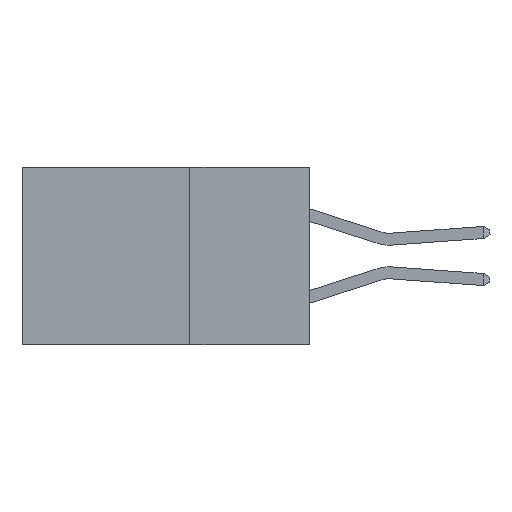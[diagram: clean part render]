
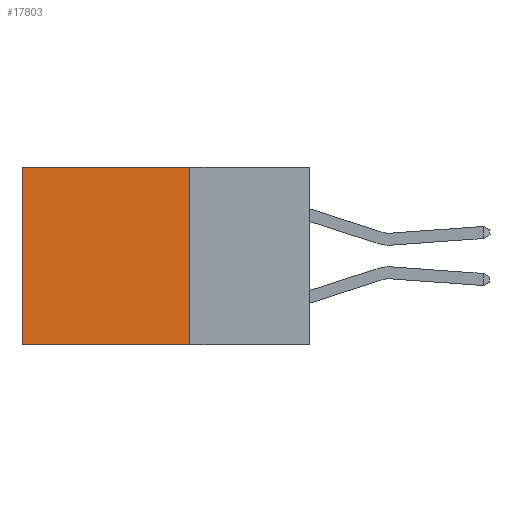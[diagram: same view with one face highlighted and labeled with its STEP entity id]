
A CAD part, left-side view. The second image highlights one B-rep face of the part: STEP entity #17803.
In plain terms, the highlighted planar face has unit normal (-1, 0, 0).
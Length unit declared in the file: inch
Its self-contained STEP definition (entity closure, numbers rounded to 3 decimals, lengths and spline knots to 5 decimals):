
#180 = VERTEX_POINT ( 'NONE', #8340 ) ;
#2442 = DIRECTION ( 'NONE',  ( 0., 1., 0. ) ) ;
#4672 = ORIENTED_EDGE ( 'NONE', *, *, #18860, .T. ) ;
#5808 = CARTESIAN_POINT ( 'NONE',  ( 0.298, 0.6, -0.37 ) ) ;
#5904 = CARTESIAN_POINT ( 'NONE',  ( 0.298, 0.6, 0. ) ) ;
#5969 = EDGE_CURVE ( 'NONE', #7264, #22438, #21239, .T. ) ;
#7264 = VERTEX_POINT ( 'NONE', #13244 ) ;
#7449 = EDGE_CURVE ( 'NONE', #7264, #180, #13951, .T. ) ;
#7457 = FACE_OUTER_BOUND ( 'NONE', #11242, .T. ) ;
#7850 = VECTOR ( 'NONE', #19917, 39.37008 ) ;
#7981 = EDGE_CURVE ( 'NONE', #180, #13580, #21459, .T. ) ;
#8331 = CARTESIAN_POINT ( 'NONE',  ( 0.298, 0.25, 0. ) ) ;
#8340 = CARTESIAN_POINT ( 'NONE',  ( 0.298, 0.25, -0.37 ) ) ;
#10156 = DIRECTION ( 'NONE',  ( 0., 0., -1. ) ) ;
#11242 = EDGE_LOOP ( 'NONE', ( #4672, #16919, #16705, #19582 ) ) ;
#11826 = DIRECTION ( 'NONE',  ( 0., 0., -1. ) ) ;
#11852 = CARTESIAN_POINT ( 'NONE',  ( 0.298, 0.25, 0. ) ) ;
#12353 = VECTOR ( 'NONE', #17952, 39.37008 ) ;
#13244 = CARTESIAN_POINT ( 'NONE',  ( 0.298, 0.25, 0. ) ) ;
#13580 = VERTEX_POINT ( 'NONE', #5808 ) ;
#13951 = LINE ( 'NONE', #11852, #18540 ) ;
#14488 = CARTESIAN_POINT ( 'NONE',  ( 0.298, 0.25, -0.37 ) ) ;
#16119 = VECTOR ( 'NONE', #2442, 39.37008 ) ;
#16128 = CARTESIAN_POINT ( 'NONE',  ( 0.298, 0.6, 0. ) ) ;
#16705 = ORIENTED_EDGE ( 'NONE', *, *, #7449, .F. ) ;
#16919 = ORIENTED_EDGE ( 'NONE', *, *, #7981, .F. ) ;
#17049 = PLANE ( 'NONE',  #21395 ) ;
#17715 = LINE ( 'NONE', #5904, #7850 ) ;
#17803 = ADVANCED_FACE ( 'NONE', ( #7457 ), #17049, .F. ) ;
#17952 = DIRECTION ( 'NONE',  ( 0., 1., 0. ) ) ;
#18540 = VECTOR ( 'NONE', #11826, 39.37008 ) ;
#18860 = EDGE_CURVE ( 'NONE', #22438, #13580, #17715, .T. ) ;
#19582 = ORIENTED_EDGE ( 'NONE', *, *, #5969, .T. ) ;
#19917 = DIRECTION ( 'NONE',  ( 0., 0., -1. ) ) ;
#20488 = DIRECTION ( 'NONE',  ( 1., 0., 0. ) ) ;
#21239 = LINE ( 'NONE', #22179, #16119 ) ;
#21395 = AXIS2_PLACEMENT_3D ( 'NONE', #8331, #20488, #10156 ) ;
#21459 = LINE ( 'NONE', #14488, #12353 ) ;
#22179 = CARTESIAN_POINT ( 'NONE',  ( 0.298, 0.25, 0. ) ) ;
#22438 = VERTEX_POINT ( 'NONE', #16128 ) ;
